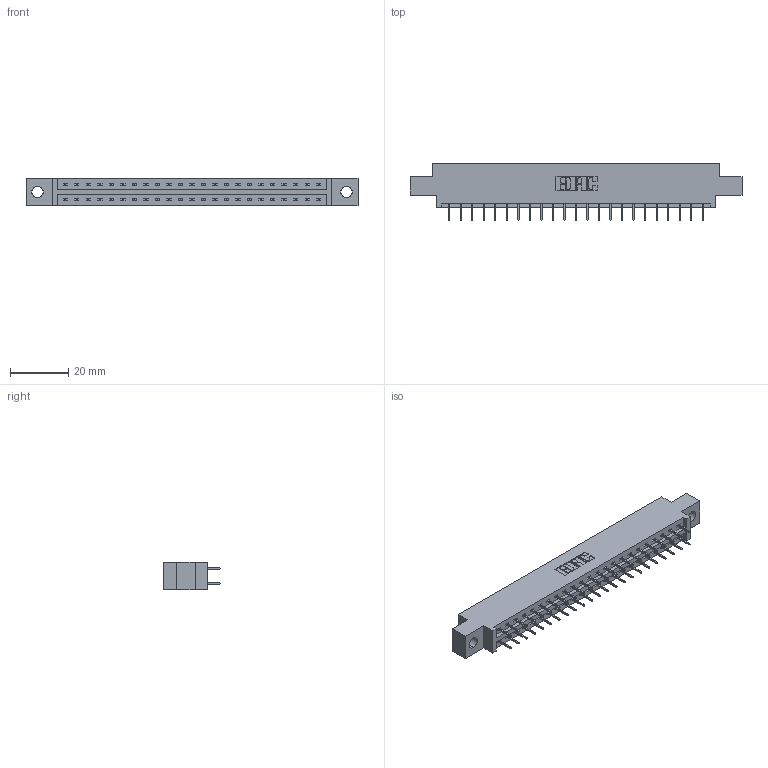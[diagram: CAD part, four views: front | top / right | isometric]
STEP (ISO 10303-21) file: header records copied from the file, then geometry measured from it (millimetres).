
FILE_DESCRIPTION (( 'STEP AP203' ), '1' );
FILE_NAME ('337-046-524-804.STEP', '2019-10-11T14:25:14', ( '' ), ( '' ), 'SwSTEP 2.0', 'SolidWorks 2016', '' );
FILE_SCHEMA (( 'CONFIG_CONTROL_DESIGN' ));
Length unit declared in the file: inch
Products named in the file (3): 337-046-524-804; 345-292-001_345-293-124; 337 Part_0.170 Offset - 0.156 Dia-TH
Assembly tree (47 placements, depth 2):
  337-046-524-804
    337 Part_0.170 Offset - 0.156 Dia-TH
    345-292-001_345-293-124  x46
Bounding box: 114.15 x 19.69 x 9.4 mm (x, y, z)
Volume: 11501.9 mm3; surface area: 12508 mm2
Topology: 47 solids, 47 shells, 2786 faces, 7913 edges, 5090 vertices
Faces by surface type: plane 2098, cylinder 688
Entity records: 20499 total; most frequent: CARTESIAN_POINT 3470, ORIENTED_EDGE 3406, DIRECTION 2987, EDGE_CURVE 1703, LINE 1579, VECTOR 1579, VERTEX_POINT 1130, AXIS2_PLACEMENT_3D 704
